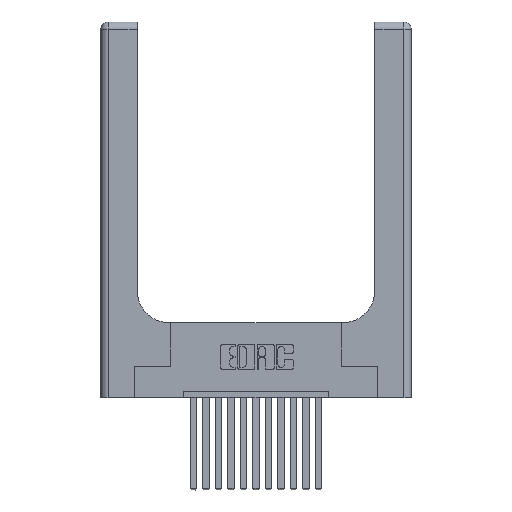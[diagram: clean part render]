
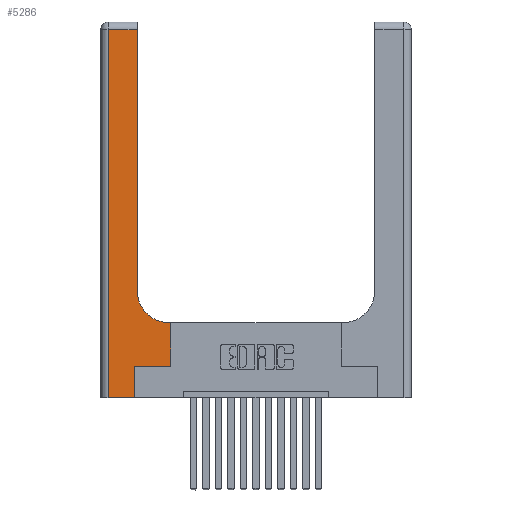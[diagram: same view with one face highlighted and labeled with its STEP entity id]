
A CAD part, top view. The second image highlights one B-rep face of the part: STEP entity #5286.
In plain terms, the highlighted planar face has unit normal (0, 0, 1).
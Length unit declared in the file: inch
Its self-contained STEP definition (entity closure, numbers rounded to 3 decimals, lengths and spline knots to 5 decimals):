
#6 = LINE ( 'NONE', #15197, #10330 ) ;
#159 = DIRECTION ( 'NONE',  ( 0., 1., 0. ) ) ;
#293 = ORIENTED_EDGE ( 'NONE', *, *, #6582, .T. ) ;
#406 = ORIENTED_EDGE ( 'NONE', *, *, #8325, .T. ) ;
#691 = ORIENTED_EDGE ( 'NONE', *, *, #10288, .T. ) ;
#929 = VERTEX_POINT ( 'NONE', #16908 ) ;
#1017 = DIRECTION ( 'NONE',  ( 1., 0., 0. ) ) ;
#1025 = LINE ( 'NONE', #15177, #9025 ) ;
#1833 = AXIS2_PLACEMENT_3D ( 'NONE', #6684, #5207, #1017 ) ;
#2112 = EDGE_CURVE ( 'NONE', #13401, #2553, #6081, .T. ) ;
#2299 = CARTESIAN_POINT ( 'NONE',  ( 0.2915, 2.94, 0.37 ) ) ;
#2369 = CARTESIAN_POINT ( 'NONE',  ( 0., 2.94, 0.37 ) ) ;
#2454 = PLANE ( 'NONE',  #2757 ) ;
#2553 = VERTEX_POINT ( 'NONE', #6107 ) ;
#2576 = CARTESIAN_POINT ( 'NONE',  ( 0.2915, 0.6, 0.37 ) ) ;
#2757 = AXIS2_PLACEMENT_3D ( 'NONE', #13381, #5181, #15948 ) ;
#3231 = FACE_OUTER_BOUND ( 'NONE', #12954, .T. ) ;
#4090 = CARTESIAN_POINT ( 'NONE',  ( 0.2915, 0.85, 0.37 ) ) ;
#4263 = CARTESIAN_POINT ( 'NONE',  ( 0.5585, 0.25, 0.37 ) ) ;
#5181 = DIRECTION ( 'NONE',  ( 0., 0., -1. ) ) ;
#5207 = DIRECTION ( 'NONE',  ( 0., 0., -1. ) ) ;
#5286 = ADVANCED_FACE ( 'NONE', ( #3231 ), #2454, .F. ) ;
#6081 = LINE ( 'NONE', #16123, #12855 ) ;
#6107 = CARTESIAN_POINT ( 'NONE',  ( 0.269, 0., 0.37 ) ) ;
#6221 = ORIENTED_EDGE ( 'NONE', *, *, #14884, .T. ) ;
#6267 = CARTESIAN_POINT ( 'NONE',  ( 0.269, 0., 0.37 ) ) ;
#6582 = EDGE_CURVE ( 'NONE', #11026, #929, #9496, .T. ) ;
#6635 = CARTESIAN_POINT ( 'NONE',  ( 0.5585, 0.6, 0.37 ) ) ;
#6669 = DIRECTION ( 'NONE',  ( -1., 0., 0. ) ) ;
#6684 = CARTESIAN_POINT ( 'NONE',  ( 0.5415, 0.85, 0.37 ) ) ;
#7089 = EDGE_CURVE ( 'NONE', #10102, #10679, #11184, .T. ) ;
#8325 = EDGE_CURVE ( 'NONE', #10219, #11026, #14139, .T. ) ;
#9025 = VECTOR ( 'NONE', #9818, 39.37008 ) ;
#9074 = VECTOR ( 'NONE', #6669, 39.37008 ) ;
#9095 = ORIENTED_EDGE ( 'NONE', *, *, #7089, .T. ) ;
#9131 = VERTEX_POINT ( 'NONE', #16580 ) ;
#9242 = DIRECTION ( 'NONE',  ( -1., 0., 0. ) ) ;
#9496 = LINE ( 'NONE', #2576, #9074 ) ;
#9662 = VECTOR ( 'NONE', #12325, 39.37008 ) ;
#9818 = DIRECTION ( 'NONE',  ( 0., -1., 0. ) ) ;
#10102 = VERTEX_POINT ( 'NONE', #4090 ) ;
#10219 = VERTEX_POINT ( 'NONE', #4263 ) ;
#10288 = EDGE_CURVE ( 'NONE', #2553, #9131, #15317, .T. ) ;
#10330 = VECTOR ( 'NONE', #14962, 39.37008 ) ;
#10533 = EDGE_CURVE ( 'NONE', #929, #10102, #11531, .T. ) ;
#10646 = ORIENTED_EDGE ( 'NONE', *, *, #13852, .T. ) ;
#10679 = VERTEX_POINT ( 'NONE', #2299 ) ;
#10732 = ORIENTED_EDGE ( 'NONE', *, *, #10533, .T. ) ;
#11026 = VERTEX_POINT ( 'NONE', #6635 ) ;
#11184 = LINE ( 'NONE', #15783, #11411 ) ;
#11411 = VECTOR ( 'NONE', #17140, 39.37008 ) ;
#11531 = CIRCLE ( 'NONE', #1833, 0.25 ) ;
#11779 = VECTOR ( 'NONE', #9242, 39.37008 ) ;
#11987 = LINE ( 'NONE', #2369, #11779 ) ;
#12325 = DIRECTION ( 'NONE',  ( 0., 1., 0. ) ) ;
#12855 = VECTOR ( 'NONE', #14639, 39.37008 ) ;
#12954 = EDGE_LOOP ( 'NONE', ( #9095, #6221, #17434, #13156, #691, #10646, #406, #293, #10732 ) ) ;
#13156 = ORIENTED_EDGE ( 'NONE', *, *, #2112, .T. ) ;
#13381 = CARTESIAN_POINT ( 'NONE',  ( 0., 3., 0.37 ) ) ;
#13401 = VERTEX_POINT ( 'NONE', #17190 ) ;
#13667 = CARTESIAN_POINT ( 'NONE',  ( 0.5585, 0.25, 0.37 ) ) ;
#13852 = EDGE_CURVE ( 'NONE', #9131, #10219, #6, .T. ) ;
#13855 = VECTOR ( 'NONE', #159, 39.37008 ) ;
#14139 = LINE ( 'NONE', #13667, #9662 ) ;
#14612 = EDGE_CURVE ( 'NONE', #17469, #13401, #1025, .T. ) ;
#14639 = DIRECTION ( 'NONE',  ( 1., 0., 0. ) ) ;
#14884 = EDGE_CURVE ( 'NONE', #10679, #17469, #11987, .T. ) ;
#14962 = DIRECTION ( 'NONE',  ( 1., 0., 0. ) ) ;
#15177 = CARTESIAN_POINT ( 'NONE',  ( 0.06, 3., 0.37 ) ) ;
#15197 = CARTESIAN_POINT ( 'NONE',  ( 0.269, 0.25, 0.37 ) ) ;
#15280 = CARTESIAN_POINT ( 'NONE',  ( 0.06, 2.94, 0.37 ) ) ;
#15317 = LINE ( 'NONE', #6267, #13855 ) ;
#15783 = CARTESIAN_POINT ( 'NONE',  ( 0.2915, 3., 0.37 ) ) ;
#15948 = DIRECTION ( 'NONE',  ( -1., 0., 0. ) ) ;
#16123 = CARTESIAN_POINT ( 'NONE',  ( 0., 0., 0.37 ) ) ;
#16580 = CARTESIAN_POINT ( 'NONE',  ( 0.269, 0.25, 0.37 ) ) ;
#16908 = CARTESIAN_POINT ( 'NONE',  ( 0.5415, 0.6, 0.37 ) ) ;
#17140 = DIRECTION ( 'NONE',  ( 0., 1., 0. ) ) ;
#17190 = CARTESIAN_POINT ( 'NONE',  ( 0.06, 0., 0.37 ) ) ;
#17434 = ORIENTED_EDGE ( 'NONE', *, *, #14612, .T. ) ;
#17469 = VERTEX_POINT ( 'NONE', #15280 ) ;
